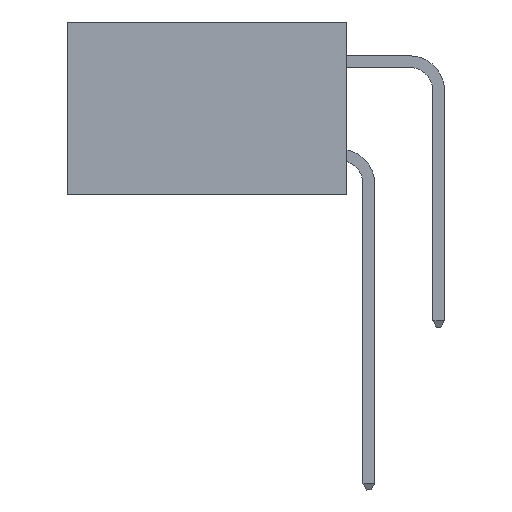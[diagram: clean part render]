
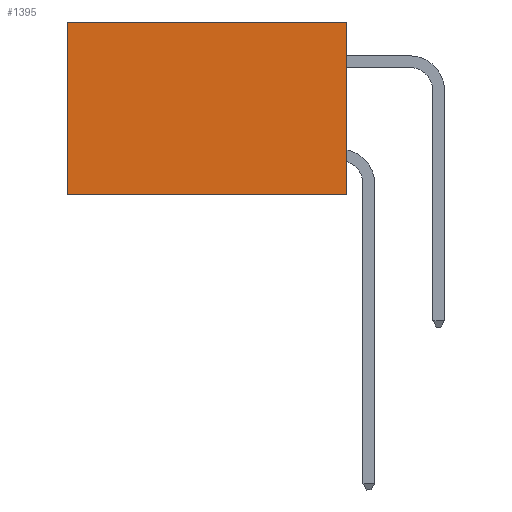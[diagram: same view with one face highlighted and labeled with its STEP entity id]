
A CAD part, left-side view. The second image highlights one B-rep face of the part: STEP entity #1395.
In plain terms, the highlighted planar face has unit normal (-1, 0, 0).
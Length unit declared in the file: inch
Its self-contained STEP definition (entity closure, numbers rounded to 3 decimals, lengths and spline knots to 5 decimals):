
#343 = AXIS2_PLACEMENT_3D ( 'NONE', #15555, #4621, #7484 ) ;
#980 = DIRECTION ( 'NONE',  ( 0., 1., 0. ) ) ;
#1238 = VERTEX_POINT ( 'NONE', #12007 ) ;
#1395 = ADVANCED_FACE ( 'NONE', ( #1859 ), #6277, .F. ) ;
#1859 = FACE_OUTER_BOUND ( 'NONE', #16018, .T. ) ;
#2145 = EDGE_CURVE ( 'NONE', #5864, #12410, #15904, .T. ) ;
#2643 = CARTESIAN_POINT ( 'NONE',  ( 0.2875, 0.6, 0. ) ) ;
#3237 = EDGE_CURVE ( 'NONE', #1238, #12410, #8084, .T. ) ;
#3467 = ORIENTED_EDGE ( 'NONE', *, *, #14459, .T. ) ;
#3775 = EDGE_CURVE ( 'NONE', #15940, #1238, #15644, .T. ) ;
#4593 = CARTESIAN_POINT ( 'NONE',  ( 0.2875, 0., 0. ) ) ;
#4621 = DIRECTION ( 'NONE',  ( 1., 0., 0. ) ) ;
#4925 = ORIENTED_EDGE ( 'NONE', *, *, #3775, .F. ) ;
#5206 = CARTESIAN_POINT ( 'NONE',  ( 0.2875, 0.6, 0. ) ) ;
#5864 = VERTEX_POINT ( 'NONE', #5206 ) ;
#6277 = PLANE ( 'NONE',  #343 ) ;
#6718 = VECTOR ( 'NONE', #980, 39.37008 ) ;
#7484 = DIRECTION ( 'NONE',  ( 0., 0., -1. ) ) ;
#7678 = VECTOR ( 'NONE', #17436, 39.37008 ) ;
#8084 = LINE ( 'NONE', #10687, #7678 ) ;
#8944 = LINE ( 'NONE', #13052, #6718 ) ;
#9542 = ORIENTED_EDGE ( 'NONE', *, *, #3237, .F. ) ;
#10181 = DIRECTION ( 'NONE',  ( 0., 0., -1. ) ) ;
#10264 = CARTESIAN_POINT ( 'NONE',  ( 0.2875, 0.6, -0.37 ) ) ;
#10687 = CARTESIAN_POINT ( 'NONE',  ( 0.2875, 0., -0.37 ) ) ;
#11579 = ORIENTED_EDGE ( 'NONE', *, *, #2145, .T. ) ;
#12007 = CARTESIAN_POINT ( 'NONE',  ( 0.2875, 0., -0.37 ) ) ;
#12410 = VERTEX_POINT ( 'NONE', #10264 ) ;
#12940 = VECTOR ( 'NONE', #16214, 39.37008 ) ;
#13052 = CARTESIAN_POINT ( 'NONE',  ( 0.2875, 0., 0. ) ) ;
#13487 = VECTOR ( 'NONE', #10181, 39.37008 ) ;
#13750 = CARTESIAN_POINT ( 'NONE',  ( 0.2875, 0., 0. ) ) ;
#14459 = EDGE_CURVE ( 'NONE', #15940, #5864, #8944, .T. ) ;
#15555 = CARTESIAN_POINT ( 'NONE',  ( 0.2875, 0., 0. ) ) ;
#15644 = LINE ( 'NONE', #13750, #13487 ) ;
#15904 = LINE ( 'NONE', #2643, #12940 ) ;
#15940 = VERTEX_POINT ( 'NONE', #4593 ) ;
#16018 = EDGE_LOOP ( 'NONE', ( #11579, #9542, #4925, #3467 ) ) ;
#16214 = DIRECTION ( 'NONE',  ( 0., 0., -1. ) ) ;
#17436 = DIRECTION ( 'NONE',  ( 0., 1., 0. ) ) ;
